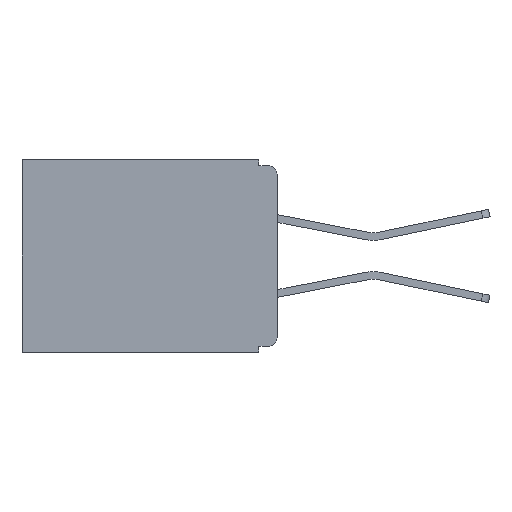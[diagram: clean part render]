
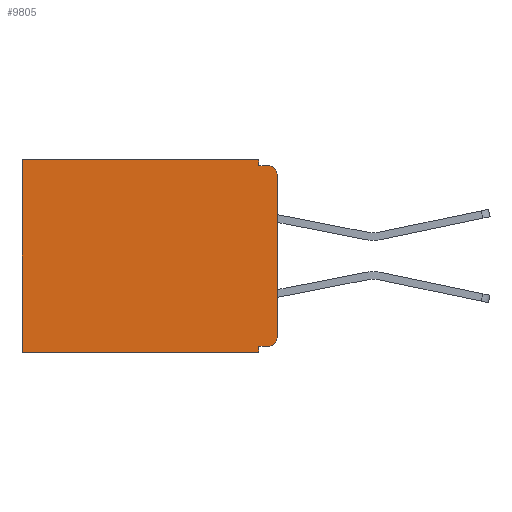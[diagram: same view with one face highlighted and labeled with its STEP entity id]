
A CAD part, left-side view. The second image highlights one B-rep face of the part: STEP entity #9805.
In plain terms, the highlighted planar face has unit normal (-1, 0, 0).
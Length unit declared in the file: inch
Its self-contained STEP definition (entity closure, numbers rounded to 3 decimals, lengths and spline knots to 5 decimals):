
#64 = DIRECTION ( 'NONE',  ( 0., 0., -1. ) ) ;
#176 = CARTESIAN_POINT ( 'NONE',  ( 0.3, 0., -0.305 ) ) ;
#544 = LINE ( 'NONE', #4349, #12744 ) ;
#751 = CIRCLE ( 'NONE', #3960, 0.015 ) ;
#953 = DIRECTION ( 'NONE',  ( 0., 0., -1. ) ) ;
#1057 = CARTESIAN_POINT ( 'NONE',  ( 0.3, 0., -0.025 ) ) ;
#1174 = EDGE_CURVE ( 'NONE', #3408, #15058, #3788, .T. ) ;
#1628 = CARTESIAN_POINT ( 'NONE',  ( 0.3, 0., -0.33 ) ) ;
#1704 = ORIENTED_EDGE ( 'NONE', *, *, #2034, .F. ) ;
#2034 = EDGE_CURVE ( 'NONE', #8464, #3190, #2066, .T. ) ;
#2066 = LINE ( 'NONE', #7463, #11008 ) ;
#2198 = VERTEX_POINT ( 'NONE', #176 ) ;
#2532 = EDGE_CURVE ( 'NONE', #18545, #8989, #544, .T. ) ;
#2699 = ORIENTED_EDGE ( 'NONE', *, *, #9062, .T. ) ;
#3190 = VERTEX_POINT ( 'NONE', #15120 ) ;
#3223 = EDGE_CURVE ( 'NONE', #5136, #15058, #751, .T. ) ;
#3408 = VERTEX_POINT ( 'NONE', #13326 ) ;
#3788 = LINE ( 'NONE', #15370, #15929 ) ;
#3950 = ORIENTED_EDGE ( 'NONE', *, *, #9833, .F. ) ;
#3960 = AXIS2_PLACEMENT_3D ( 'NONE', #9190, #9436, #10270 ) ;
#3972 = ORIENTED_EDGE ( 'NONE', *, *, #2532, .F. ) ;
#4135 = VECTOR ( 'NONE', #953, 39.37008 ) ;
#4349 = CARTESIAN_POINT ( 'NONE',  ( 0.3, 0., -0.32 ) ) ;
#4581 = CARTESIAN_POINT ( 'NONE',  ( 0.3, 0.031, -0.33 ) ) ;
#4635 = DIRECTION ( 'NONE',  ( 0., -1., 0. ) ) ;
#5136 = VERTEX_POINT ( 'NONE', #1057 ) ;
#5216 = ORIENTED_EDGE ( 'NONE', *, *, #11543, .F. ) ;
#5720 = EDGE_CURVE ( 'NONE', #8989, #8464, #19522, .T. ) ;
#5969 = PLANE ( 'NONE',  #17138 ) ;
#6430 = DIRECTION ( 'NONE',  ( 0., 0., -1. ) ) ;
#6947 = VERTEX_POINT ( 'NONE', #8858 ) ;
#7224 = AXIS2_PLACEMENT_3D ( 'NONE', #17537, #8046, #19133 ) ;
#7282 = VECTOR ( 'NONE', #11765, 39.37008 ) ;
#7383 = DIRECTION ( 'NONE',  ( 0., 1., 0. ) ) ;
#7463 = CARTESIAN_POINT ( 'NONE',  ( 0.3, 0., -0.33 ) ) ;
#7768 = LINE ( 'NONE', #11838, #7282 ) ;
#8046 = DIRECTION ( 'NONE',  ( -1., 0., 0. ) ) ;
#8063 = CARTESIAN_POINT ( 'NONE',  ( 0.3, 0., -0.33 ) ) ;
#8065 = CARTESIAN_POINT ( 'NONE',  ( 0.3, 0.031, -0.33 ) ) ;
#8397 = LINE ( 'NONE', #9487, #20506 ) ;
#8464 = VERTEX_POINT ( 'NONE', #4581 ) ;
#8634 = ORIENTED_EDGE ( 'NONE', *, *, #12240, .T. ) ;
#8858 = CARTESIAN_POINT ( 'NONE',  ( 0.3, 0.031, 0. ) ) ;
#8989 = VERTEX_POINT ( 'NONE', #13493 ) ;
#9062 = EDGE_CURVE ( 'NONE', #6947, #9170, #7768, .T. ) ;
#9170 = VERTEX_POINT ( 'NONE', #11157 ) ;
#9190 = CARTESIAN_POINT ( 'NONE',  ( 0.3, 0.015, -0.025 ) ) ;
#9436 = DIRECTION ( 'NONE',  ( -1., 0., 0. ) ) ;
#9487 = CARTESIAN_POINT ( 'NONE',  ( 0.3, 0.031, 0. ) ) ;
#9624 = DIRECTION ( 'NONE',  ( 1., 0., 0. ) ) ;
#9805 = ADVANCED_FACE ( 'NONE', ( #20092 ), #5969, .F. ) ;
#9833 = EDGE_CURVE ( 'NONE', #5136, #2198, #15444, .T. ) ;
#10155 = ORIENTED_EDGE ( 'NONE', *, *, #5720, .F. ) ;
#10270 = DIRECTION ( 'NONE',  ( 0., 0., -1. ) ) ;
#11008 = VECTOR ( 'NONE', #7383, 39.37008 ) ;
#11131 = ORIENTED_EDGE ( 'NONE', *, *, #20539, .T. ) ;
#11157 = CARTESIAN_POINT ( 'NONE',  ( 0.3, 0.437, 0. ) ) ;
#11356 = ORIENTED_EDGE ( 'NONE', *, *, #3223, .T. ) ;
#11543 = EDGE_CURVE ( 'NONE', #6947, #3408, #8397, .T. ) ;
#11765 = DIRECTION ( 'NONE',  ( 0., 1., 0. ) ) ;
#11838 = CARTESIAN_POINT ( 'NONE',  ( 0.3, 0., 0. ) ) ;
#11844 = CIRCLE ( 'NONE', #7224, 0.015 ) ;
#12240 = EDGE_CURVE ( 'NONE', #18545, #2198, #11844, .T. ) ;
#12553 = LINE ( 'NONE', #19922, #4135 ) ;
#12744 = VECTOR ( 'NONE', #12894, 39.37008 ) ;
#12757 = EDGE_LOOP ( 'NONE', ( #3950, #11356, #20513, #5216, #2699, #11131, #1704, #10155, #3972, #8634 ) ) ;
#12894 = DIRECTION ( 'NONE',  ( 0., 1., 0. ) ) ;
#13326 = CARTESIAN_POINT ( 'NONE',  ( 0.3, 0.031, -0.01 ) ) ;
#13493 = CARTESIAN_POINT ( 'NONE',  ( 0.3, 0.031, -0.32 ) ) ;
#15058 = VERTEX_POINT ( 'NONE', #18893 ) ;
#15120 = CARTESIAN_POINT ( 'NONE',  ( 0.3, 0.437, -0.33 ) ) ;
#15346 = VECTOR ( 'NONE', #17627, 39.37008 ) ;
#15370 = CARTESIAN_POINT ( 'NONE',  ( 0.3, 0., -0.01 ) ) ;
#15444 = LINE ( 'NONE', #8063, #19130 ) ;
#15929 = VECTOR ( 'NONE', #4635, 39.37008 ) ;
#17138 = AXIS2_PLACEMENT_3D ( 'NONE', #1628, #9624, #64 ) ;
#17296 = DIRECTION ( 'NONE',  ( 0., 0., -1. ) ) ;
#17537 = CARTESIAN_POINT ( 'NONE',  ( 0.3, 0.015, -0.305 ) ) ;
#17627 = DIRECTION ( 'NONE',  ( 0., 0., -1. ) ) ;
#18545 = VERTEX_POINT ( 'NONE', #19390 ) ;
#18893 = CARTESIAN_POINT ( 'NONE',  ( 0.3, 0.015, -0.01 ) ) ;
#19130 = VECTOR ( 'NONE', #6430, 39.37008 ) ;
#19133 = DIRECTION ( 'NONE',  ( 0., 0., -1. ) ) ;
#19390 = CARTESIAN_POINT ( 'NONE',  ( 0.3, 0.015, -0.32 ) ) ;
#19522 = LINE ( 'NONE', #8065, #15346 ) ;
#19922 = CARTESIAN_POINT ( 'NONE',  ( 0.3, 0.437, -0.33 ) ) ;
#20092 = FACE_OUTER_BOUND ( 'NONE', #12757, .T. ) ;
#20506 = VECTOR ( 'NONE', #17296, 39.37008 ) ;
#20513 = ORIENTED_EDGE ( 'NONE', *, *, #1174, .F. ) ;
#20539 = EDGE_CURVE ( 'NONE', #9170, #3190, #12553, .T. ) ;
